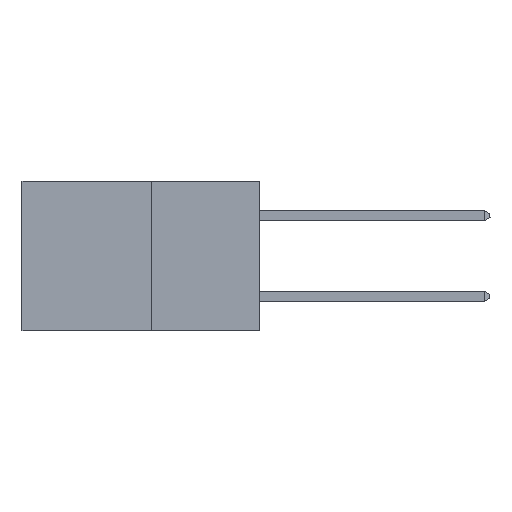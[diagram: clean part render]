
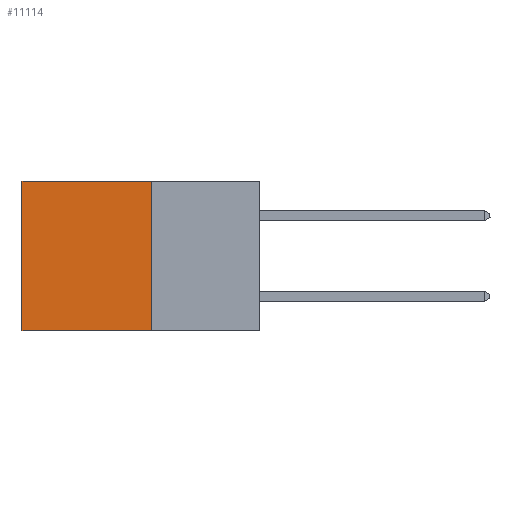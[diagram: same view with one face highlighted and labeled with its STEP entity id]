
A CAD part, left-side view. The second image highlights one B-rep face of the part: STEP entity #11114.
In plain terms, the highlighted planar face has unit normal (-1, 0, 0).
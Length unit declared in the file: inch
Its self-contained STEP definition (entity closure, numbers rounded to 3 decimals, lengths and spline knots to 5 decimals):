
#509 = LINE ( 'NONE', #3042, #33129 ) ;
#1553 = EDGE_CURVE ( 'NONE', #32178, #14005, #509, .T. ) ;
#1689 = ORIENTED_EDGE ( 'NONE', *, *, #1553, .T. ) ;
#2054 = DIRECTION ( 'NONE',  ( 0., 0., -1. ) ) ;
#2352 = CARTESIAN_POINT ( 'NONE',  ( 0.277, 0.59, -0.37 ) ) ;
#2434 = LINE ( 'NONE', #13315, #29728 ) ;
#3042 = CARTESIAN_POINT ( 'NONE',  ( 0.277, 0.27, 0. ) ) ;
#7301 = VECTOR ( 'NONE', #12617, 39.37008 ) ;
#8719 = EDGE_CURVE ( 'NONE', #32178, #12567, #17557, .T. ) ;
#10928 = ORIENTED_EDGE ( 'NONE', *, *, #8719, .F. ) ;
#11114 = ADVANCED_FACE ( 'NONE', ( #32617 ), #12542, .F. ) ;
#11817 = LINE ( 'NONE', #28492, #7301 ) ;
#11958 = ORIENTED_EDGE ( 'NONE', *, *, #21155, .F. ) ;
#12542 = PLANE ( 'NONE',  #29899 ) ;
#12567 = VERTEX_POINT ( 'NONE', #15241 ) ;
#12617 = DIRECTION ( 'NONE',  ( 0., 1., 0. ) ) ;
#13315 = CARTESIAN_POINT ( 'NONE',  ( 0.277, 0.59, -0.37 ) ) ;
#13424 = ORIENTED_EDGE ( 'NONE', *, *, #25595, .T. ) ;
#14005 = VERTEX_POINT ( 'NONE', #24721 ) ;
#14810 = DIRECTION ( 'NONE',  ( 0., 1., 0. ) ) ;
#15213 = CARTESIAN_POINT ( 'NONE',  ( 0.277, 0.27, -0.37 ) ) ;
#15241 = CARTESIAN_POINT ( 'NONE',  ( 0.277, 0.27, -0.37 ) ) ;
#17557 = LINE ( 'NONE', #28235, #30758 ) ;
#17926 = DIRECTION ( 'NONE',  ( 1., 0., 0. ) ) ;
#20544 = CARTESIAN_POINT ( 'NONE',  ( 0.277, 0.27, 0. ) ) ;
#21155 = EDGE_CURVE ( 'NONE', #12567, #21282, #11817, .T. ) ;
#21282 = VERTEX_POINT ( 'NONE', #2352 ) ;
#21430 = DIRECTION ( 'NONE',  ( 0., 0., -1. ) ) ;
#24721 = CARTESIAN_POINT ( 'NONE',  ( 0.277, 0.59, 0. ) ) ;
#25595 = EDGE_CURVE ( 'NONE', #14005, #21282, #2434, .T. ) ;
#28235 = CARTESIAN_POINT ( 'NONE',  ( 0.277, 0.27, -0.37 ) ) ;
#28492 = CARTESIAN_POINT ( 'NONE',  ( 0.277, 0.27, -0.37 ) ) ;
#29204 = EDGE_LOOP ( 'NONE', ( #13424, #11958, #10928, #1689 ) ) ;
#29728 = VECTOR ( 'NONE', #21430, 39.37008 ) ;
#29899 = AXIS2_PLACEMENT_3D ( 'NONE', #15213, #17926, #2054 ) ;
#30758 = VECTOR ( 'NONE', #30880, 39.37008 ) ;
#30880 = DIRECTION ( 'NONE',  ( 0., 0., -1. ) ) ;
#32178 = VERTEX_POINT ( 'NONE', #20544 ) ;
#32617 = FACE_OUTER_BOUND ( 'NONE', #29204, .T. ) ;
#33129 = VECTOR ( 'NONE', #14810, 39.37008 ) ;
